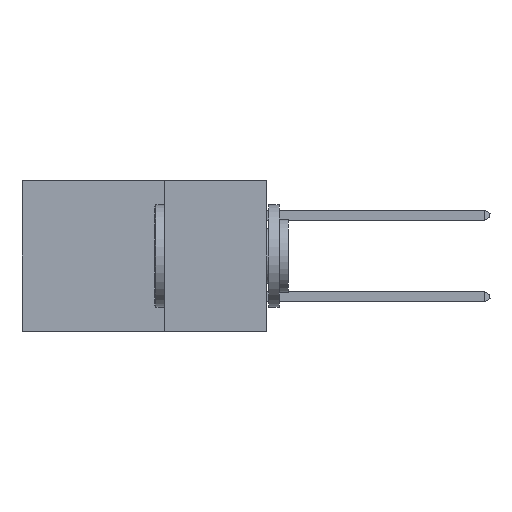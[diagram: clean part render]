
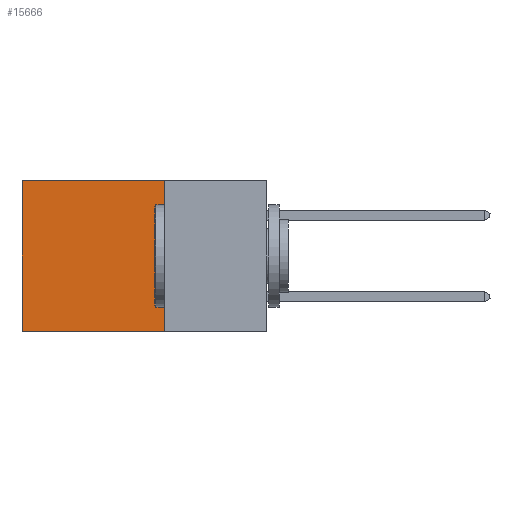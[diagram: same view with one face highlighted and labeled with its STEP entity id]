
A CAD part, left-side view. The second image highlights one B-rep face of the part: STEP entity #15666.
In plain terms, the highlighted planar face has unit normal (-1, 0, 0).
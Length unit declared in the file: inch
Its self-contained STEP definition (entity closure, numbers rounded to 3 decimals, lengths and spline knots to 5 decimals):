
#812 = LINE ( 'NONE', #37640, #3580 ) ;
#2539 = LINE ( 'NONE', #21723, #6238 ) ;
#2560 = CARTESIAN_POINT ( 'NONE',  ( 0.2875, 0.25, 0. ) ) ;
#3153 = EDGE_CURVE ( 'NONE', #6607, #6218, #812, .T. ) ;
#3580 = VECTOR ( 'NONE', #22677, 39.37008 ) ;
#3591 = DIRECTION ( 'NONE',  ( 0., 1., 0. ) ) ;
#5237 = ORIENTED_EDGE ( 'NONE', *, *, #37329, .T. ) ;
#6218 = VERTEX_POINT ( 'NONE', #18023 ) ;
#6238 = VECTOR ( 'NONE', #27539, 39.37008 ) ;
#6607 = VERTEX_POINT ( 'NONE', #2560 ) ;
#7181 = CARTESIAN_POINT ( 'NONE',  ( 0.2875, 0.6, 0. ) ) ;
#10089 = DIRECTION ( 'NONE',  ( 0., 1., 0. ) ) ;
#11287 = LINE ( 'NONE', #28170, #17782 ) ;
#13352 = VERTEX_POINT ( 'NONE', #24309 ) ;
#13797 = FACE_OUTER_BOUND ( 'NONE', #37737, .T. ) ;
#15666 = ADVANCED_FACE ( 'NONE', ( #13797 ), #31394, .F. ) ;
#15685 = LINE ( 'NONE', #30445, #37842 ) ;
#16839 = ORIENTED_EDGE ( 'NONE', *, *, #28370, .F. ) ;
#17782 = VECTOR ( 'NONE', #10089, 39.37008 ) ;
#18023 = CARTESIAN_POINT ( 'NONE',  ( 0.2875, 0.25, -0.37 ) ) ;
#19194 = VERTEX_POINT ( 'NONE', #7181 ) ;
#19254 = DIRECTION ( 'NONE',  ( 0., 0., -1. ) ) ;
#19638 = DIRECTION ( 'NONE',  ( 1., 0., 0. ) ) ;
#21723 = CARTESIAN_POINT ( 'NONE',  ( 0.2875, 0.6, 0. ) ) ;
#22677 = DIRECTION ( 'NONE',  ( 0., 0., -1. ) ) ;
#24309 = CARTESIAN_POINT ( 'NONE',  ( 0.2875, 0.6, -0.37 ) ) ;
#27539 = DIRECTION ( 'NONE',  ( 0., 0., -1. ) ) ;
#28170 = CARTESIAN_POINT ( 'NONE',  ( 0.2875, 0.25, 0. ) ) ;
#28370 = EDGE_CURVE ( 'NONE', #6218, #13352, #15685, .T. ) ;
#29912 = AXIS2_PLACEMENT_3D ( 'NONE', #36938, #19638, #19254 ) ;
#30445 = CARTESIAN_POINT ( 'NONE',  ( 0.2875, 0.25, -0.37 ) ) ;
#31394 = PLANE ( 'NONE',  #29912 ) ;
#32242 = ORIENTED_EDGE ( 'NONE', *, *, #3153, .F. ) ;
#36938 = CARTESIAN_POINT ( 'NONE',  ( 0.2875, 0.25, 0. ) ) ;
#37038 = EDGE_CURVE ( 'NONE', #19194, #13352, #2539, .T. ) ;
#37329 = EDGE_CURVE ( 'NONE', #6607, #19194, #11287, .T. ) ;
#37640 = CARTESIAN_POINT ( 'NONE',  ( 0.2875, 0.25, 0. ) ) ;
#37737 = EDGE_LOOP ( 'NONE', ( #38031, #16839, #32242, #5237 ) ) ;
#37842 = VECTOR ( 'NONE', #3591, 39.37008 ) ;
#38031 = ORIENTED_EDGE ( 'NONE', *, *, #37038, .T. ) ;
